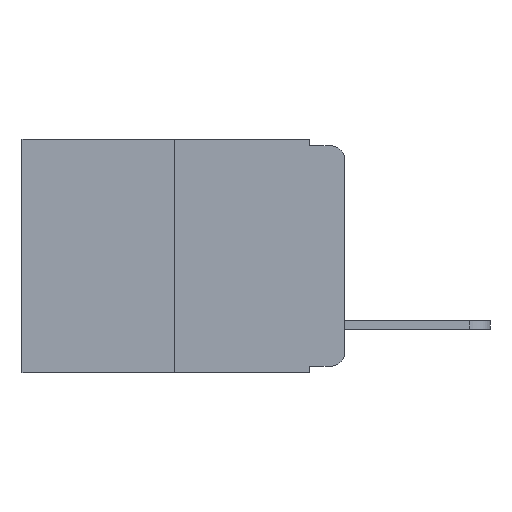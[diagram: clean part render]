
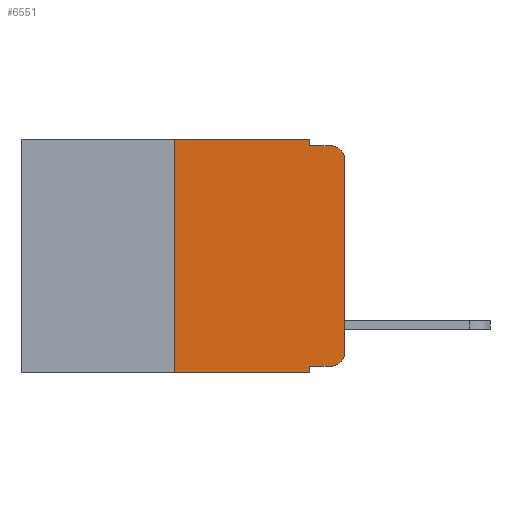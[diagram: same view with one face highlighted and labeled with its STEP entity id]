
A CAD part, left-side view. The second image highlights one B-rep face of the part: STEP entity #6551.
In plain terms, the highlighted planar face has unit normal (-1, 0, 0).
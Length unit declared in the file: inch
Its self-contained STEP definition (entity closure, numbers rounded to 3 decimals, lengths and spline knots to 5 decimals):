
#398 = DIRECTION ( 'NONE',  ( 0., 0., -1. ) ) ;
#705 = LINE ( 'NONE', #15973, #10395 ) ;
#758 = LINE ( 'NONE', #5873, #19950 ) ;
#768 = CIRCLE ( 'NONE', #16555, 0.02 ) ;
#925 = VERTEX_POINT ( 'NONE', #18389 ) ;
#1194 = DIRECTION ( 'NONE',  ( 0., 0., -1. ) ) ;
#1872 = CARTESIAN_POINT ( 'NONE',  ( 0., 0.051, -0.333 ) ) ;
#2267 = VECTOR ( 'NONE', #1194, 39.37008 ) ;
#3069 = LINE ( 'NONE', #16157, #7559 ) ;
#3763 = EDGE_CURVE ( 'NONE', #15345, #16870, #10280, .T. ) ;
#4773 = AXIS2_PLACEMENT_3D ( 'NONE', #13774, #13745, #13713 ) ;
#5344 = LINE ( 'NONE', #19554, #19309 ) ;
#5708 = VERTEX_POINT ( 'NONE', #17677 ) ;
#5873 = CARTESIAN_POINT ( 'NONE',  ( 0., 0., 0. ) ) ;
#5955 = EDGE_LOOP ( 'NONE', ( #8798, #14589, #9379, #9638, #14530, #10332, #12199, #11896, #13933, #12489 ) ) ;
#6294 = EDGE_CURVE ( 'NONE', #12844, #16870, #23255, .T. ) ;
#6551 = ADVANCED_FACE ( 'NONE', ( #21467 ), #8905, .F. ) ;
#6989 = DIRECTION ( 'NONE',  ( 0., -1., 0. ) ) ;
#7176 = CARTESIAN_POINT ( 'NONE',  ( 0., 0.25, 0. ) ) ;
#7473 = VERTEX_POINT ( 'NONE', #19565 ) ;
#7557 = EDGE_CURVE ( 'NONE', #16860, #12844, #758, .T. ) ;
#7559 = VECTOR ( 'NONE', #6989, 39.37008 ) ;
#8352 = EDGE_CURVE ( 'NONE', #21327, #9458, #705, .T. ) ;
#8773 = DIRECTION ( 'NONE',  ( 0., 0., -1. ) ) ;
#8796 = DIRECTION ( 'NONE',  ( 1., 0., 0. ) ) ;
#8798 = ORIENTED_EDGE ( 'NONE', *, *, #7557, .T. ) ;
#8799 = CARTESIAN_POINT ( 'NONE',  ( 0., 0.473, 0. ) ) ;
#8905 = PLANE ( 'NONE',  #21295 ) ;
#9073 = LINE ( 'NONE', #7176, #22588 ) ;
#9379 = ORIENTED_EDGE ( 'NONE', *, *, #3763, .F. ) ;
#9458 = VERTEX_POINT ( 'NONE', #19840 ) ;
#9638 = ORIENTED_EDGE ( 'NONE', *, *, #23379, .F. ) ;
#10280 = LINE ( 'NONE', #19241, #10908 ) ;
#10332 = ORIENTED_EDGE ( 'NONE', *, *, #20138, .F. ) ;
#10395 = VECTOR ( 'NONE', #14585, 39.37008 ) ;
#10908 = VECTOR ( 'NONE', #19238, 39.37008 ) ;
#11565 = CARTESIAN_POINT ( 'NONE',  ( 0., 0.051, -0.01 ) ) ;
#11896 = ORIENTED_EDGE ( 'NONE', *, *, #17779, .F. ) ;
#11976 = DIRECTION ( 'NONE',  ( -1., 0., 0. ) ) ;
#12199 = ORIENTED_EDGE ( 'NONE', *, *, #23066, .T. ) ;
#12232 = CARTESIAN_POINT ( 'NONE',  ( 0., 0.25, 0. ) ) ;
#12489 = ORIENTED_EDGE ( 'NONE', *, *, #13094, .T. ) ;
#12844 = VERTEX_POINT ( 'NONE', #21521 ) ;
#12927 = VERTEX_POINT ( 'NONE', #1872 ) ;
#13066 = CARTESIAN_POINT ( 'NONE',  ( 0., 0.02, -0.01 ) ) ;
#13094 = EDGE_CURVE ( 'NONE', #5708, #16860, #768, .T. ) ;
#13713 = DIRECTION ( 'NONE',  ( 0., 0., -1. ) ) ;
#13745 = DIRECTION ( 'NONE',  ( -1., 0., 0. ) ) ;
#13774 = CARTESIAN_POINT ( 'NONE',  ( 0., 0.02, -0.03 ) ) ;
#13933 = ORIENTED_EDGE ( 'NONE', *, *, #16621, .T. ) ;
#14530 = ORIENTED_EDGE ( 'NONE', *, *, #8352, .F. ) ;
#14585 = DIRECTION ( 'NONE',  ( 0., -1., 0. ) ) ;
#14589 = ORIENTED_EDGE ( 'NONE', *, *, #6294, .T. ) ;
#14812 = CARTESIAN_POINT ( 'NONE',  ( 0., 0., -0.313 ) ) ;
#15345 = VERTEX_POINT ( 'NONE', #11565 ) ;
#15973 = CARTESIAN_POINT ( 'NONE',  ( 0., 0.473, 0. ) ) ;
#16157 = CARTESIAN_POINT ( 'NONE',  ( 0., 0.473, -0.343 ) ) ;
#16555 = AXIS2_PLACEMENT_3D ( 'NONE', #22346, #11976, #398 ) ;
#16621 = EDGE_CURVE ( 'NONE', #12927, #5708, #5344, .T. ) ;
#16860 = VERTEX_POINT ( 'NONE', #14812 ) ;
#16870 = VERTEX_POINT ( 'NONE', #13066 ) ;
#17127 = LINE ( 'NONE', #21333, #2267 ) ;
#17677 = CARTESIAN_POINT ( 'NONE',  ( 0., 0.02, -0.333 ) ) ;
#17779 = EDGE_CURVE ( 'NONE', #12927, #925, #17127, .T. ) ;
#18389 = CARTESIAN_POINT ( 'NONE',  ( 0., 0.051, -0.343 ) ) ;
#18510 = CARTESIAN_POINT ( 'NONE',  ( 0., 0.051, 0. ) ) ;
#19238 = DIRECTION ( 'NONE',  ( 0., -1., 0. ) ) ;
#19241 = CARTESIAN_POINT ( 'NONE',  ( 0., 0.051, -0.01 ) ) ;
#19309 = VECTOR ( 'NONE', #21222, 39.37008 ) ;
#19554 = CARTESIAN_POINT ( 'NONE',  ( 0., 0.051, -0.333 ) ) ;
#19565 = CARTESIAN_POINT ( 'NONE',  ( 0., 0.25, -0.343 ) ) ;
#19765 = DIRECTION ( 'NONE',  ( 0., 0., 1. ) ) ;
#19840 = CARTESIAN_POINT ( 'NONE',  ( 0., 0.051, 0. ) ) ;
#19950 = VECTOR ( 'NONE', #20694, 39.37008 ) ;
#20138 = EDGE_CURVE ( 'NONE', #7473, #21327, #9073, .T. ) ;
#20257 = DIRECTION ( 'NONE',  ( 0., 0., -1. ) ) ;
#20513 = VECTOR ( 'NONE', #20257, 39.37008 ) ;
#20694 = DIRECTION ( 'NONE',  ( 0., 0., 1. ) ) ;
#21013 = LINE ( 'NONE', #18510, #20513 ) ;
#21222 = DIRECTION ( 'NONE',  ( 0., -1., 0. ) ) ;
#21295 = AXIS2_PLACEMENT_3D ( 'NONE', #8799, #8796, #8773 ) ;
#21327 = VERTEX_POINT ( 'NONE', #12232 ) ;
#21333 = CARTESIAN_POINT ( 'NONE',  ( 0., 0.051, 0. ) ) ;
#21467 = FACE_OUTER_BOUND ( 'NONE', #5955, .T. ) ;
#21521 = CARTESIAN_POINT ( 'NONE',  ( 0., 0., -0.03 ) ) ;
#22346 = CARTESIAN_POINT ( 'NONE',  ( 0., 0.02, -0.313 ) ) ;
#22588 = VECTOR ( 'NONE', #19765, 39.37008 ) ;
#23066 = EDGE_CURVE ( 'NONE', #7473, #925, #3069, .T. ) ;
#23255 = CIRCLE ( 'NONE', #4773, 0.02 ) ;
#23379 = EDGE_CURVE ( 'NONE', #9458, #15345, #21013, .T. ) ;
